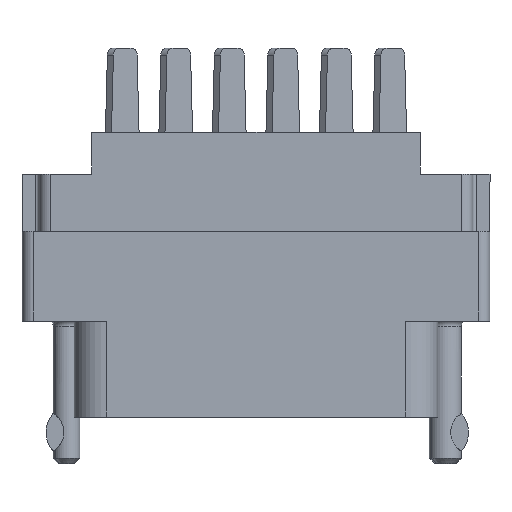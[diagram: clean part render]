
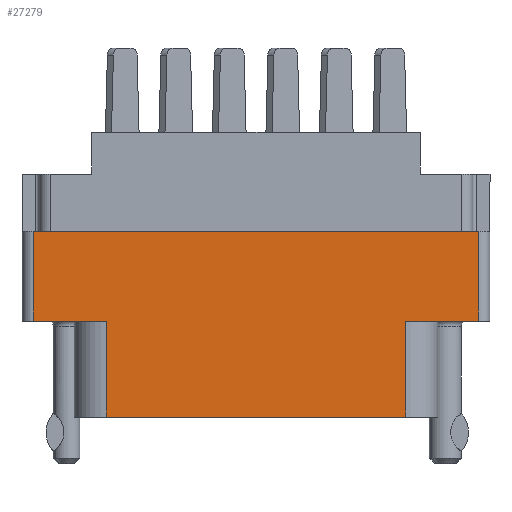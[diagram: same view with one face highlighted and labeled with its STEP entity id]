
A CAD part, front view. The second image highlights one B-rep face of the part: STEP entity #27279.
In plain terms, the highlighted planar face has unit normal (0, -1, 0).
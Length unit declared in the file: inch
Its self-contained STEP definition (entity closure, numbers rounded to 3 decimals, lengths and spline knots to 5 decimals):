
#18 = LINE ( 'NONE', #25996, #16088 ) ;
#44 = DIRECTION ( 'NONE',  ( 0., 0., -1. ) ) ;
#470 = VERTEX_POINT ( 'NONE', #30589 ) ;
#596 = VERTEX_POINT ( 'NONE', #13615 ) ;
#4316 = EDGE_CURVE ( 'NONE', #25913, #29201, #6169, .T. ) ;
#5346 = CARTESIAN_POINT ( 'NONE',  ( 0.42, -0.343, -0.798 ) ) ;
#6169 = LINE ( 'NONE', #26712, #21551 ) ;
#6201 = VERTEX_POINT ( 'NONE', #8940 ) ;
#6554 = VERTEX_POINT ( 'NONE', #30558 ) ;
#8940 = CARTESIAN_POINT ( 'NONE',  ( 0.624, -0.343, -0.277 ) ) ;
#10010 = LINE ( 'NONE', #23561, #32297 ) ;
#10512 = ORIENTED_EDGE ( 'NONE', *, *, #12218, .F. ) ;
#10937 = DIRECTION ( 'NONE',  ( 0., 0., -1. ) ) ;
#11046 = DIRECTION ( 'NONE',  ( 1., 0., 0. ) ) ;
#11716 = EDGE_CURVE ( 'NONE', #24256, #6201, #30749, .T. ) ;
#11898 = DIRECTION ( 'NONE',  ( -1., 0., 0. ) ) ;
#12218 = EDGE_CURVE ( 'NONE', #24256, #25913, #17499, .T. ) ;
#12641 = VECTOR ( 'NONE', #17209, 39.37008 ) ;
#13615 = CARTESIAN_POINT ( 'NONE',  ( -0.624, -0.343, -0.529 ) ) ;
#14511 = ORIENTED_EDGE ( 'NONE', *, *, #22899, .F. ) ;
#14564 = DIRECTION ( 'NONE',  ( 1., 0., 0. ) ) ;
#14735 = LINE ( 'NONE', #16767, #26405 ) ;
#15366 = LINE ( 'NONE', #17579, #28497 ) ;
#16001 = DIRECTION ( 'NONE',  ( 0., 0., 1. ) ) ;
#16023 = EDGE_CURVE ( 'NONE', #32682, #29201, #14735, .T. ) ;
#16088 = VECTOR ( 'NONE', #11046, 39.37008 ) ;
#16196 = ORIENTED_EDGE ( 'NONE', *, *, #26434, .F. ) ;
#16767 = CARTESIAN_POINT ( 'NONE',  ( -0.624, -0.343, -0.798 ) ) ;
#17209 = DIRECTION ( 'NONE',  ( 0., 0., 1. ) ) ;
#17499 = LINE ( 'NONE', #22414, #29976 ) ;
#17579 = CARTESIAN_POINT ( 'NONE',  ( -0.656, -0.343, -0.277 ) ) ;
#17907 = DIRECTION ( 'NONE',  ( 1., 0., 0. ) ) ;
#18368 = VECTOR ( 'NONE', #16001, 39.37008 ) ;
#18382 = LINE ( 'NONE', #28717, #18368 ) ;
#18552 = FACE_OUTER_BOUND ( 'NONE', #24803, .T. ) ;
#18711 = DIRECTION ( 'NONE',  ( 0., -1., 0. ) ) ;
#20565 = AXIS2_PLACEMENT_3D ( 'NONE', #31095, #18711, #44 ) ;
#20780 = PLANE ( 'NONE',  #20565 ) ;
#20854 = EDGE_CURVE ( 'NONE', #6554, #32682, #10010, .T. ) ;
#20956 = ORIENTED_EDGE ( 'NONE', *, *, #4316, .F. ) ;
#21551 = VECTOR ( 'NONE', #10937, 39.37008 ) ;
#22023 = CARTESIAN_POINT ( 'NONE',  ( 0.42, -0.343, -0.529 ) ) ;
#22414 = CARTESIAN_POINT ( 'NONE',  ( 0., -0.343, -0.529 ) ) ;
#22417 = CARTESIAN_POINT ( 'NONE',  ( 0.624, -0.343, -0.529 ) ) ;
#22899 = EDGE_CURVE ( 'NONE', #470, #6201, #15366, .T. ) ;
#23243 = DIRECTION ( 'NONE',  ( 0., 0., -1. ) ) ;
#23561 = CARTESIAN_POINT ( 'NONE',  ( -0.42, -0.343, -0.529 ) ) ;
#23975 = EDGE_CURVE ( 'NONE', #596, #6554, #18, .T. ) ;
#24256 = VERTEX_POINT ( 'NONE', #22417 ) ;
#24803 = EDGE_LOOP ( 'NONE', ( #26195, #26122, #20956, #10512, #26498, #14511, #16196, #33194 ) ) ;
#25351 = CARTESIAN_POINT ( 'NONE',  ( 0.624, -0.343, -0.798 ) ) ;
#25913 = VERTEX_POINT ( 'NONE', #22023 ) ;
#25996 = CARTESIAN_POINT ( 'NONE',  ( 0., -0.343, -0.529 ) ) ;
#26122 = ORIENTED_EDGE ( 'NONE', *, *, #16023, .T. ) ;
#26195 = ORIENTED_EDGE ( 'NONE', *, *, #20854, .T. ) ;
#26405 = VECTOR ( 'NONE', #14564, 39.37008 ) ;
#26434 = EDGE_CURVE ( 'NONE', #596, #470, #18382, .T. ) ;
#26498 = ORIENTED_EDGE ( 'NONE', *, *, #11716, .T. ) ;
#26712 = CARTESIAN_POINT ( 'NONE',  ( 0.42, -0.343, -0.529 ) ) ;
#27279 = ADVANCED_FACE ( 'NONE', ( #18552 ), #20780, .T. ) ;
#28497 = VECTOR ( 'NONE', #17907, 39.37008 ) ;
#28717 = CARTESIAN_POINT ( 'NONE',  ( -0.624, -0.343, -0.798 ) ) ;
#29201 = VERTEX_POINT ( 'NONE', #5346 ) ;
#29976 = VECTOR ( 'NONE', #11898, 39.37008 ) ;
#30558 = CARTESIAN_POINT ( 'NONE',  ( -0.42, -0.343, -0.529 ) ) ;
#30589 = CARTESIAN_POINT ( 'NONE',  ( -0.624, -0.343, -0.277 ) ) ;
#30749 = LINE ( 'NONE', #25351, #12641 ) ;
#30868 = CARTESIAN_POINT ( 'NONE',  ( -0.42, -0.343, -0.798 ) ) ;
#31095 = CARTESIAN_POINT ( 'NONE',  ( -0.624, -0.343, -0.798 ) ) ;
#32297 = VECTOR ( 'NONE', #23243, 39.37008 ) ;
#32682 = VERTEX_POINT ( 'NONE', #30868 ) ;
#33194 = ORIENTED_EDGE ( 'NONE', *, *, #23975, .T. ) ;
